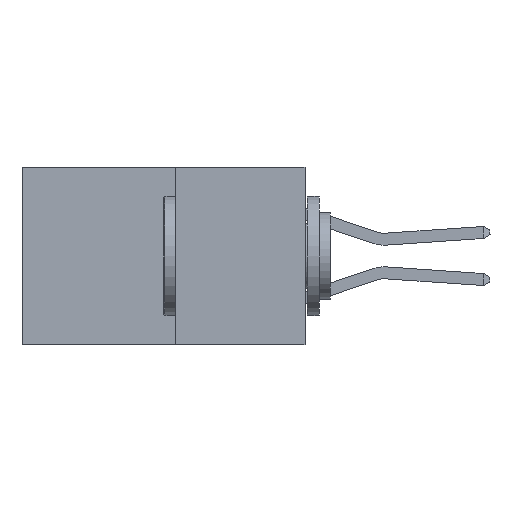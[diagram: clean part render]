
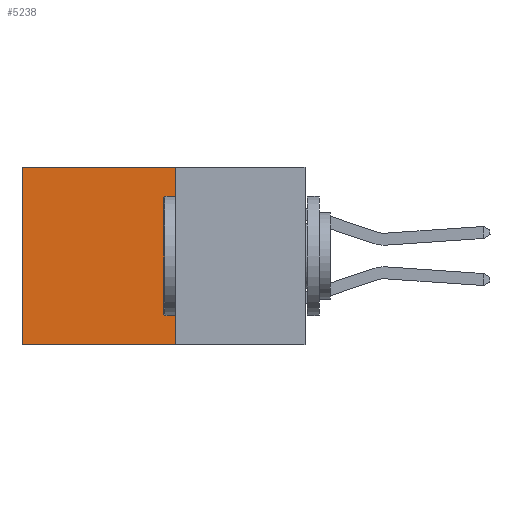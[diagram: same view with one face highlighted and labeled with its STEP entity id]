
A CAD part, left-side view. The second image highlights one B-rep face of the part: STEP entity #5238.
In plain terms, the highlighted planar face has unit normal (-1, 0, 0).
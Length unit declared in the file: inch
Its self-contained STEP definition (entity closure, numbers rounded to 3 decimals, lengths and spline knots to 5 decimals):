
#852 = ORIENTED_EDGE ( 'NONE', *, *, #14129, .F. ) ;
#1463 = ORIENTED_EDGE ( 'NONE', *, *, #9041, .F. ) ;
#1981 = LINE ( 'NONE', #2312, #14429 ) ;
#2270 = DIRECTION ( 'NONE',  ( 0., 1., 0. ) ) ;
#2312 = CARTESIAN_POINT ( 'NONE',  ( 0.277, 0.27, -0.37 ) ) ;
#2711 = VECTOR ( 'NONE', #5492, 39.37008 ) ;
#2742 = DIRECTION ( 'NONE',  ( 0., 0., -1. ) ) ;
#3283 = VERTEX_POINT ( 'NONE', #6445 ) ;
#3636 = EDGE_CURVE ( 'NONE', #3283, #13253, #14643, .T. ) ;
#3855 = LINE ( 'NONE', #8450, #19707 ) ;
#4216 = CARTESIAN_POINT ( 'NONE',  ( 0.277, 0.27, -0.37 ) ) ;
#4247 = EDGE_LOOP ( 'NONE', ( #14202, #1463, #852, #16138 ) ) ;
#4801 = CARTESIAN_POINT ( 'NONE',  ( 0.277, 0.59, -0.37 ) ) ;
#5237 = VECTOR ( 'NONE', #2742, 39.37008 ) ;
#5238 = ADVANCED_FACE ( 'NONE', ( #7850 ), #10565, .F. ) ;
#5492 = DIRECTION ( 'NONE',  ( 0., 0., -1. ) ) ;
#5764 = VERTEX_POINT ( 'NONE', #15362 ) ;
#6052 = AXIS2_PLACEMENT_3D ( 'NONE', #11431, #11425, #11415 ) ;
#6445 = CARTESIAN_POINT ( 'NONE',  ( 0.277, 0.59, 0. ) ) ;
#6931 = CARTESIAN_POINT ( 'NONE',  ( 0.277, 0.59, -0.37 ) ) ;
#7850 = FACE_OUTER_BOUND ( 'NONE', #4247, .T. ) ;
#8450 = CARTESIAN_POINT ( 'NONE',  ( 0.277, 0.27, 0. ) ) ;
#8475 = DIRECTION ( 'NONE',  ( 0., 1., 0. ) ) ;
#9041 = EDGE_CURVE ( 'NONE', #5764, #13253, #1981, .T. ) ;
#10565 = PLANE ( 'NONE',  #6052 ) ;
#10792 = EDGE_CURVE ( 'NONE', #12533, #3283, #3855, .T. ) ;
#11415 = DIRECTION ( 'NONE',  ( 0., 0., -1. ) ) ;
#11425 = DIRECTION ( 'NONE',  ( 1., 0., 0. ) ) ;
#11431 = CARTESIAN_POINT ( 'NONE',  ( 0.277, 0.27, -0.37 ) ) ;
#12533 = VERTEX_POINT ( 'NONE', #13189 ) ;
#13189 = CARTESIAN_POINT ( 'NONE',  ( 0.277, 0.27, 0. ) ) ;
#13253 = VERTEX_POINT ( 'NONE', #6931 ) ;
#13547 = LINE ( 'NONE', #4216, #5237 ) ;
#14129 = EDGE_CURVE ( 'NONE', #12533, #5764, #13547, .T. ) ;
#14202 = ORIENTED_EDGE ( 'NONE', *, *, #3636, .T. ) ;
#14429 = VECTOR ( 'NONE', #2270, 39.37008 ) ;
#14643 = LINE ( 'NONE', #4801, #2711 ) ;
#15362 = CARTESIAN_POINT ( 'NONE',  ( 0.277, 0.27, -0.37 ) ) ;
#16138 = ORIENTED_EDGE ( 'NONE', *, *, #10792, .T. ) ;
#19707 = VECTOR ( 'NONE', #8475, 39.37008 ) ;
